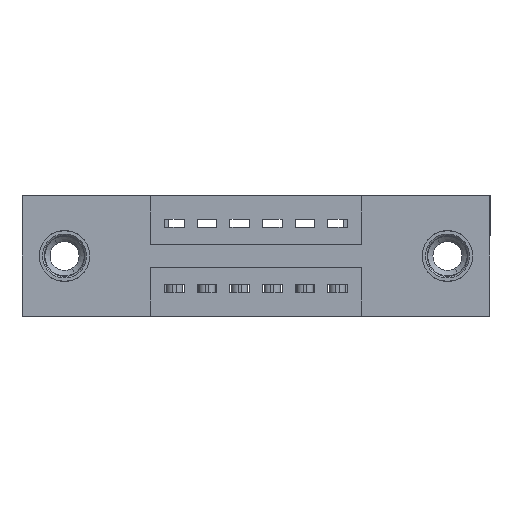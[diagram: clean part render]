
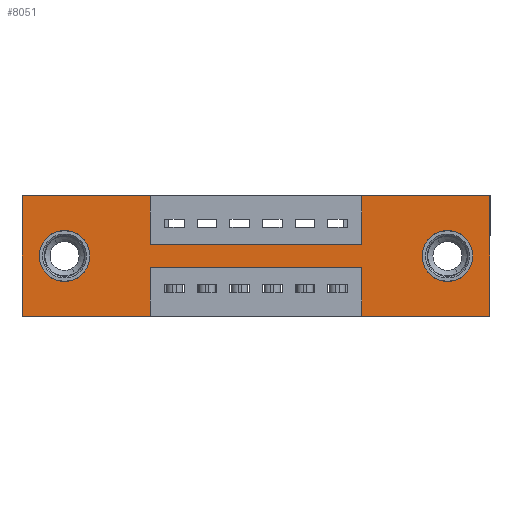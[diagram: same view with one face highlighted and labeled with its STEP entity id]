
A CAD part, front view. The second image highlights one B-rep face of the part: STEP entity #8051.
In plain terms, the highlighted planar face has unit normal (0, -1, 0).
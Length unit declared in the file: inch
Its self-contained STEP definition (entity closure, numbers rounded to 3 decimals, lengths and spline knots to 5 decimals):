
#145 = CARTESIAN_POINT ( 'NONE',  ( 0., 0., -0.37 ) ) ;
#166 = CARTESIAN_POINT ( 'NONE',  ( 0., 0., 0. ) ) ;
#185 = LINE ( 'NONE', #5439, #5957 ) ;
#365 = EDGE_CURVE ( 'NONE', #13761, #10685, #9529, .T. ) ;
#368 = EDGE_CURVE ( 'NONE', #599, #1161, #1052, .T. ) ;
#456 = CARTESIAN_POINT ( 'NONE',  ( 1.0425, 0., -0.37 ) ) ;
#508 = ORIENTED_EDGE ( 'NONE', *, *, #9957, .F. ) ;
#583 = CARTESIAN_POINT ( 'NONE',  ( 0.13, 0., -0.185 ) ) ;
#599 = VERTEX_POINT ( 'NONE', #10643 ) ;
#738 = DIRECTION ( 'NONE',  ( 0., 0., 1. ) ) ;
#864 = CARTESIAN_POINT ( 'NONE',  ( 1.0425, 0., 0. ) ) ;
#1052 = CIRCLE ( 'NONE', #10657, 0.078 ) ;
#1137 = VERTEX_POINT ( 'NONE', #5226 ) ;
#1161 = VERTEX_POINT ( 'NONE', #8380 ) ;
#1198 = VECTOR ( 'NONE', #10992, 39.37008 ) ;
#1332 = DIRECTION ( 'NONE',  ( -1., 0., 0. ) ) ;
#1341 = DIRECTION ( 'NONE',  ( 0., 0., 1. ) ) ;
#1409 = CARTESIAN_POINT ( 'NONE',  ( 1.305, 0., -0.263 ) ) ;
#1529 = ORIENTED_EDGE ( 'NONE', *, *, #1652, .F. ) ;
#1646 = ORIENTED_EDGE ( 'NONE', *, *, #8896, .F. ) ;
#1652 = EDGE_CURVE ( 'NONE', #9021, #12441, #2710, .T. ) ;
#1725 = CARTESIAN_POINT ( 'NONE',  ( 0., 0., -0.37 ) ) ;
#1967 = CARTESIAN_POINT ( 'NONE',  ( 1.305, 0., -0.185 ) ) ;
#1985 = CIRCLE ( 'NONE', #12371, 0.078 ) ;
#2128 = EDGE_CURVE ( 'NONE', #4555, #6414, #12730, .T. ) ;
#2317 = CARTESIAN_POINT ( 'NONE',  ( 0.3925, 0., 0. ) ) ;
#2385 = LINE ( 'NONE', #166, #2884 ) ;
#2498 = CARTESIAN_POINT ( 'NONE',  ( 0., 0., -0.37 ) ) ;
#2583 = ORIENTED_EDGE ( 'NONE', *, *, #2837, .F. ) ;
#2618 = DIRECTION ( 'NONE',  ( 0., 0., -1. ) ) ;
#2710 = LINE ( 'NONE', #7070, #7944 ) ;
#2815 = DIRECTION ( 'NONE',  ( 0., 1., 0. ) ) ;
#2837 = EDGE_CURVE ( 'NONE', #1137, #4555, #7112, .T. ) ;
#2884 = VECTOR ( 'NONE', #1341, 39.37008 ) ;
#3094 = LINE ( 'NONE', #6029, #6665 ) ;
#3188 = ORIENTED_EDGE ( 'NONE', *, *, #9877, .F. ) ;
#3216 = EDGE_LOOP ( 'NONE', ( #9593, #7723 ) ) ;
#3404 = CARTESIAN_POINT ( 'NONE',  ( 0., 0., 0. ) ) ;
#3467 = EDGE_CURVE ( 'NONE', #12441, #1137, #4705, .T. ) ;
#3523 = VECTOR ( 'NONE', #9075, 39.37008 ) ;
#3990 = DIRECTION ( 'NONE',  ( 0., 1., 0. ) ) ;
#4002 = VECTOR ( 'NONE', #6198, 39.37008 ) ;
#4186 = VECTOR ( 'NONE', #1332, 39.37008 ) ;
#4478 = FACE_BOUND ( 'NONE', #8773, .T. ) ;
#4555 = VERTEX_POINT ( 'NONE', #10789 ) ;
#4644 = DIRECTION ( 'NONE',  ( 0., 1., 0. ) ) ;
#4689 = EDGE_CURVE ( 'NONE', #1161, #599, #1985, .T. ) ;
#4696 = ORIENTED_EDGE ( 'NONE', *, *, #13680, .T. ) ;
#4705 = LINE ( 'NONE', #11422, #3523 ) ;
#4774 = DIRECTION ( 'NONE',  ( -1., 0., 0. ) ) ;
#4854 = DIRECTION ( 'NONE',  ( -1., 0., 0. ) ) ;
#5189 = VERTEX_POINT ( 'NONE', #12879 ) ;
#5226 = CARTESIAN_POINT ( 'NONE',  ( 1.0425, 0., -0.15 ) ) ;
#5439 = CARTESIAN_POINT ( 'NONE',  ( 0.3925, 0., -0.37 ) ) ;
#5490 = ORIENTED_EDGE ( 'NONE', *, *, #8394, .T. ) ;
#5522 = VERTEX_POINT ( 'NONE', #3404 ) ;
#5821 = CARTESIAN_POINT ( 'NONE',  ( 0., 0., -0.37 ) ) ;
#5865 = CARTESIAN_POINT ( 'NONE',  ( 0.3925, 0., -0.15 ) ) ;
#5957 = VECTOR ( 'NONE', #11990, 39.37008 ) ;
#5987 = DIRECTION ( 'NONE',  ( 0., 0., 1. ) ) ;
#6029 = CARTESIAN_POINT ( 'NONE',  ( 1.0425, 0., -0.37 ) ) ;
#6055 = DIRECTION ( 'NONE',  ( 0., 0., -1. ) ) ;
#6198 = DIRECTION ( 'NONE',  ( 1., 0., 0. ) ) ;
#6383 = EDGE_CURVE ( 'NONE', #5522, #9021, #10101, .T. ) ;
#6414 = VERTEX_POINT ( 'NONE', #13478 ) ;
#6546 = LINE ( 'NONE', #145, #4186 ) ;
#6662 = VECTOR ( 'NONE', #4854, 39.37008 ) ;
#6665 = VECTOR ( 'NONE', #5987, 39.37008 ) ;
#6946 = VECTOR ( 'NONE', #12967, 39.37008 ) ;
#7021 = DIRECTION ( 'NONE',  ( 0., 0., -1. ) ) ;
#7070 = CARTESIAN_POINT ( 'NONE',  ( 0.3925, 0., 0. ) ) ;
#7112 = LINE ( 'NONE', #864, #6946 ) ;
#7320 = DIRECTION ( 'NONE',  ( 0., 0., -1. ) ) ;
#7723 = ORIENTED_EDGE ( 'NONE', *, *, #368, .T. ) ;
#7841 = CIRCLE ( 'NONE', #9197, 0.078 ) ;
#7929 = VERTEX_POINT ( 'NONE', #5821 ) ;
#7944 = VECTOR ( 'NONE', #2618, 39.37008 ) ;
#8009 = VERTEX_POINT ( 'NONE', #1409 ) ;
#8010 = VERTEX_POINT ( 'NONE', #456 ) ;
#8051 = ADVANCED_FACE ( 'NONE', ( #4478, #12107, #9206 ), #8975, .T. ) ;
#8291 = ORIENTED_EDGE ( 'NONE', *, *, #2128, .F. ) ;
#8318 = CARTESIAN_POINT ( 'NONE',  ( 0.3925, 0., -0.37 ) ) ;
#8380 = CARTESIAN_POINT ( 'NONE',  ( 0.13, 0., -0.107 ) ) ;
#8394 = EDGE_CURVE ( 'NONE', #8009, #5189, #7841, .T. ) ;
#8773 = EDGE_LOOP ( 'NONE', ( #4696, #5490 ) ) ;
#8896 = EDGE_CURVE ( 'NONE', #8010, #13761, #3094, .T. ) ;
#8975 = PLANE ( 'NONE',  #9901 ) ;
#8998 = ORIENTED_EDGE ( 'NONE', *, *, #9337, .F. ) ;
#9021 = VERTEX_POINT ( 'NONE', #2317 ) ;
#9075 = DIRECTION ( 'NONE',  ( 1., 0., 0. ) ) ;
#9139 = DIRECTION ( 'NONE',  ( 0., 0., 1. ) ) ;
#9197 = AXIS2_PLACEMENT_3D ( 'NONE', #11137, #4644, #12239 ) ;
#9206 = FACE_OUTER_BOUND ( 'NONE', #11925, .T. ) ;
#9337 = EDGE_CURVE ( 'NONE', #10685, #9398, #185, .T. ) ;
#9348 = CARTESIAN_POINT ( 'NONE',  ( 1.435, 0., -0.37 ) ) ;
#9398 = VERTEX_POINT ( 'NONE', #8318 ) ;
#9529 = LINE ( 'NONE', #10266, #6662 ) ;
#9593 = ORIENTED_EDGE ( 'NONE', *, *, #4689, .T. ) ;
#9791 = LINE ( 'NONE', #10244, #12542 ) ;
#9877 = EDGE_CURVE ( 'NONE', #7929, #5522, #2385, .T. ) ;
#9894 = CARTESIAN_POINT ( 'NONE',  ( 0., 0., 0. ) ) ;
#9901 = AXIS2_PLACEMENT_3D ( 'NONE', #2498, #10072, #6055 ) ;
#9957 = EDGE_CURVE ( 'NONE', #13140, #8010, #10009, .T. ) ;
#10009 = LINE ( 'NONE', #1725, #10358 ) ;
#10072 = DIRECTION ( 'NONE',  ( 0., -1., 0. ) ) ;
#10101 = LINE ( 'NONE', #13836, #4002 ) ;
#10244 = CARTESIAN_POINT ( 'NONE',  ( 1.435, 0., 0. ) ) ;
#10266 = CARTESIAN_POINT ( 'NONE',  ( 0.3925, 0., -0.22 ) ) ;
#10358 = VECTOR ( 'NONE', #4774, 39.37008 ) ;
#10643 = CARTESIAN_POINT ( 'NONE',  ( 0.13, 0., -0.263 ) ) ;
#10657 = AXIS2_PLACEMENT_3D ( 'NONE', #11508, #2815, #738 ) ;
#10685 = VERTEX_POINT ( 'NONE', #11210 ) ;
#10789 = CARTESIAN_POINT ( 'NONE',  ( 1.0425, 0., 0. ) ) ;
#10957 = CIRCLE ( 'NONE', #12444, 0.078 ) ;
#10992 = DIRECTION ( 'NONE',  ( 1., 0., 0. ) ) ;
#11137 = CARTESIAN_POINT ( 'NONE',  ( 1.305, 0., -0.185 ) ) ;
#11210 = CARTESIAN_POINT ( 'NONE',  ( 0.3925, 0., -0.22 ) ) ;
#11237 = ORIENTED_EDGE ( 'NONE', *, *, #6383, .F. ) ;
#11313 = ORIENTED_EDGE ( 'NONE', *, *, #11481, .F. ) ;
#11422 = CARTESIAN_POINT ( 'NONE',  ( 0.3925, 0., -0.15 ) ) ;
#11438 = DIRECTION ( 'NONE',  ( 0., 1., 0. ) ) ;
#11481 = EDGE_CURVE ( 'NONE', #6414, #13140, #9791, .T. ) ;
#11508 = CARTESIAN_POINT ( 'NONE',  ( 0.13, 0., -0.185 ) ) ;
#11925 = EDGE_LOOP ( 'NONE', ( #8998, #12499, #1646, #508, #11313, #8291, #2583, #13137, #1529, #11237, #3188, #12647 ) ) ;
#11990 = DIRECTION ( 'NONE',  ( 0., 0., -1. ) ) ;
#12107 = FACE_BOUND ( 'NONE', #3216, .T. ) ;
#12239 = DIRECTION ( 'NONE',  ( 0., 0., -1. ) ) ;
#12371 = AXIS2_PLACEMENT_3D ( 'NONE', #583, #11438, #9139 ) ;
#12441 = VERTEX_POINT ( 'NONE', #5865 ) ;
#12444 = AXIS2_PLACEMENT_3D ( 'NONE', #1967, #3990, #7320 ) ;
#12499 = ORIENTED_EDGE ( 'NONE', *, *, #365, .F. ) ;
#12542 = VECTOR ( 'NONE', #7021, 39.37008 ) ;
#12647 = ORIENTED_EDGE ( 'NONE', *, *, #13875, .F. ) ;
#12730 = LINE ( 'NONE', #9894, #1198 ) ;
#12879 = CARTESIAN_POINT ( 'NONE',  ( 1.305, 0., -0.107 ) ) ;
#12967 = DIRECTION ( 'NONE',  ( 0., 0., 1. ) ) ;
#12969 = CARTESIAN_POINT ( 'NONE',  ( 1.0425, 0., -0.22 ) ) ;
#13137 = ORIENTED_EDGE ( 'NONE', *, *, #3467, .F. ) ;
#13140 = VERTEX_POINT ( 'NONE', #9348 ) ;
#13478 = CARTESIAN_POINT ( 'NONE',  ( 1.435, 0., 0. ) ) ;
#13680 = EDGE_CURVE ( 'NONE', #5189, #8009, #10957, .T. ) ;
#13761 = VERTEX_POINT ( 'NONE', #12969 ) ;
#13836 = CARTESIAN_POINT ( 'NONE',  ( 0., 0., 0. ) ) ;
#13875 = EDGE_CURVE ( 'NONE', #9398, #7929, #6546, .T. ) ;
